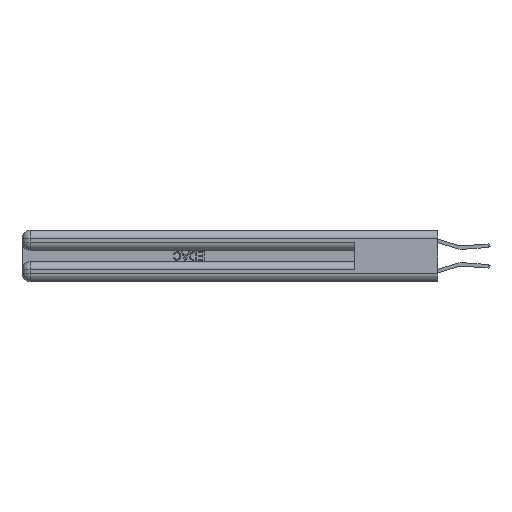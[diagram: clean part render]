
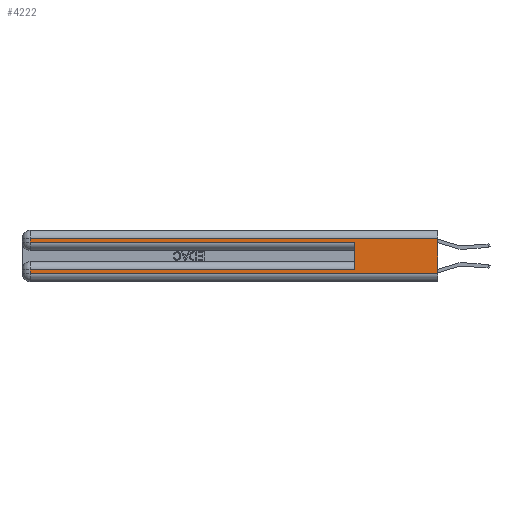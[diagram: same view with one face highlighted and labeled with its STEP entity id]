
A CAD part, left-side view. The second image highlights one B-rep face of the part: STEP entity #4222.
In plain terms, the highlighted planar face has unit normal (-1, 0, 0).
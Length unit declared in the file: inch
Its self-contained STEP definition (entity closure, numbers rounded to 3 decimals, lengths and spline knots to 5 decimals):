
#18 = DIRECTION ( 'NONE',  ( 0., 0., -1. ) ) ;
#110 = DIRECTION ( 'NONE',  ( 0., 1., 0. ) ) ;
#114 = CARTESIAN_POINT ( 'NONE',  ( 0., 2.94, 0.085 ) ) ;
#203 = EDGE_CURVE ( 'NONE', #15077, #15820, #319, .T. ) ;
#319 = LINE ( 'NONE', #11181, #27033 ) ;
#514 = CARTESIAN_POINT ( 'NONE',  ( 0., 0.6, 0.145 ) ) ;
#766 = VERTEX_POINT ( 'NONE', #3761 ) ;
#896 = LINE ( 'NONE', #11617, #4381 ) ;
#2112 = EDGE_CURVE ( 'NONE', #4648, #14379, #6553, .T. ) ;
#2323 = ORIENTED_EDGE ( 'NONE', *, *, #2112, .T. ) ;
#2918 = ORIENTED_EDGE ( 'NONE', *, *, #8387, .T. ) ;
#3683 = AXIS2_PLACEMENT_3D ( 'NONE', #10596, #12981, #18 ) ;
#3761 = CARTESIAN_POINT ( 'NONE',  ( 0., 2.94, 0.285 ) ) ;
#3865 = DIRECTION ( 'NONE',  ( 0., 0., -1. ) ) ;
#4083 = CARTESIAN_POINT ( 'NONE',  ( 0., 2.94, 0.06 ) ) ;
#4222 = ADVANCED_FACE ( 'NONE', ( #17514 ), #23752, .F. ) ;
#4381 = VECTOR ( 'NONE', #5547, 39.37008 ) ;
#4465 = VECTOR ( 'NONE', #13040, 39.37008 ) ;
#4648 = VERTEX_POINT ( 'NONE', #4083 ) ;
#5453 = VERTEX_POINT ( 'NONE', #19564 ) ;
#5547 = DIRECTION ( 'NONE',  ( 0., 0., -1. ) ) ;
#5688 = EDGE_CURVE ( 'NONE', #15820, #4648, #23076, .T. ) ;
#5710 = ORIENTED_EDGE ( 'NONE', *, *, #5688, .T. ) ;
#6184 = EDGE_CURVE ( 'NONE', #5453, #16969, #21583, .T. ) ;
#6388 = CARTESIAN_POINT ( 'NONE',  ( 0., 0., 0.37 ) ) ;
#6553 = LINE ( 'NONE', #6687, #4465 ) ;
#6687 = CARTESIAN_POINT ( 'NONE',  ( 0., 0., 0.06 ) ) ;
#7107 = VECTOR ( 'NONE', #21985, 39.37008 ) ;
#7427 = LINE ( 'NONE', #514, #7107 ) ;
#7950 = CARTESIAN_POINT ( 'NONE',  ( 0., 2.94, 0.37 ) ) ;
#8227 = DIRECTION ( 'NONE',  ( 0., -1., 0. ) ) ;
#8304 = CARTESIAN_POINT ( 'NONE',  ( 0., 2.94, 0.31 ) ) ;
#8387 = EDGE_CURVE ( 'NONE', #766, #22190, #19260, .T. ) ;
#9052 = ORIENTED_EDGE ( 'NONE', *, *, #11405, .F. ) ;
#9210 = VECTOR ( 'NONE', #8227, 39.37008 ) ;
#9373 = ORIENTED_EDGE ( 'NONE', *, *, #22524, .T. ) ;
#10596 = CARTESIAN_POINT ( 'NONE',  ( 0., 0., 0.37 ) ) ;
#10831 = CARTESIAN_POINT ( 'NONE',  ( 0., 0., 0.31 ) ) ;
#11181 = CARTESIAN_POINT ( 'NONE',  ( 0., 0., 0.085 ) ) ;
#11405 = EDGE_CURVE ( 'NONE', #15077, #22190, #7427, .T. ) ;
#11617 = CARTESIAN_POINT ( 'NONE',  ( 0., 2.94, 0.37 ) ) ;
#11980 = CARTESIAN_POINT ( 'NONE',  ( 0., 0., 0.06 ) ) ;
#12981 = DIRECTION ( 'NONE',  ( 1., 0., 0. ) ) ;
#13040 = DIRECTION ( 'NONE',  ( 0., -1., 0. ) ) ;
#14379 = VERTEX_POINT ( 'NONE', #11980 ) ;
#14633 = CARTESIAN_POINT ( 'NONE',  ( 0., 0.6, 0.085 ) ) ;
#15077 = VERTEX_POINT ( 'NONE', #14633 ) ;
#15681 = ORIENTED_EDGE ( 'NONE', *, *, #6184, .T. ) ;
#15703 = DIRECTION ( 'NONE',  ( 0., 1., 0. ) ) ;
#15820 = VERTEX_POINT ( 'NONE', #114 ) ;
#16969 = VERTEX_POINT ( 'NONE', #8304 ) ;
#17405 = LINE ( 'NONE', #6388, #18869 ) ;
#17514 = FACE_OUTER_BOUND ( 'NONE', #26774, .T. ) ;
#18869 = VECTOR ( 'NONE', #23784, 39.37008 ) ;
#19260 = LINE ( 'NONE', #27932, #9210 ) ;
#19463 = EDGE_CURVE ( 'NONE', #5453, #14379, #17405, .T. ) ;
#19564 = CARTESIAN_POINT ( 'NONE',  ( 0., 0., 0.31 ) ) ;
#19575 = VECTOR ( 'NONE', #110, 39.37008 ) ;
#20694 = VECTOR ( 'NONE', #3865, 39.37008 ) ;
#21583 = LINE ( 'NONE', #10831, #19575 ) ;
#21985 = DIRECTION ( 'NONE',  ( 0., 0., 1. ) ) ;
#22190 = VERTEX_POINT ( 'NONE', #23367 ) ;
#22524 = EDGE_CURVE ( 'NONE', #16969, #766, #896, .T. ) ;
#23076 = LINE ( 'NONE', #7950, #20694 ) ;
#23367 = CARTESIAN_POINT ( 'NONE',  ( 0., 0.6, 0.285 ) ) ;
#23752 = PLANE ( 'NONE',  #3683 ) ;
#23784 = DIRECTION ( 'NONE',  ( 0., 0., -1. ) ) ;
#25691 = ORIENTED_EDGE ( 'NONE', *, *, #203, .T. ) ;
#26709 = ORIENTED_EDGE ( 'NONE', *, *, #19463, .F. ) ;
#26774 = EDGE_LOOP ( 'NONE', ( #26709, #15681, #9373, #2918, #9052, #25691, #5710, #2323 ) ) ;
#27033 = VECTOR ( 'NONE', #15703, 39.37008 ) ;
#27932 = CARTESIAN_POINT ( 'NONE',  ( 0., 0., 0.285 ) ) ;
